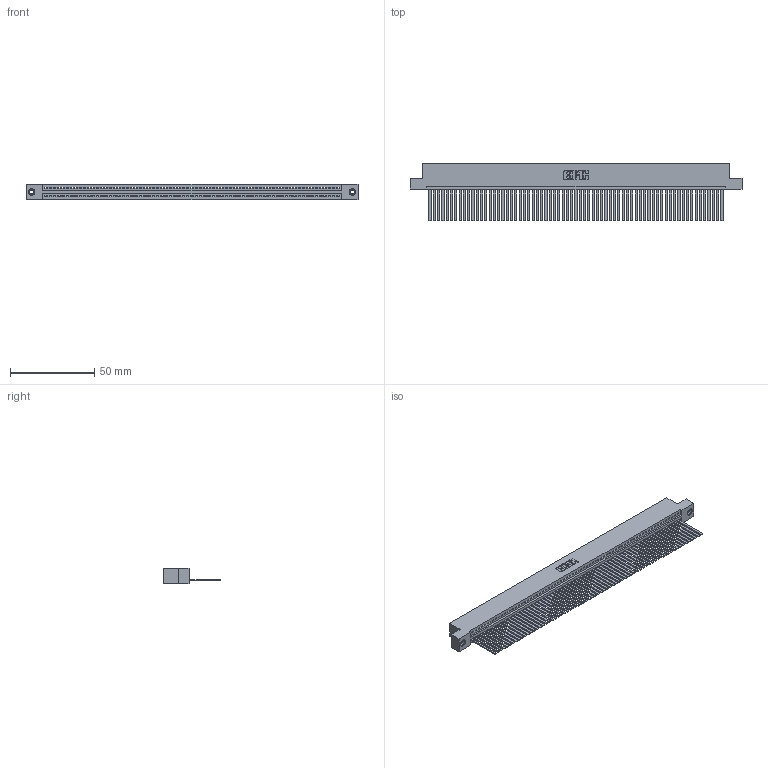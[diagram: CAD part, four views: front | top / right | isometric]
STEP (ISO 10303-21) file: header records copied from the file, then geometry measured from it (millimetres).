
FILE_DESCRIPTION (( 'STEP AP203' ), '1' );
FILE_NAME ('345-069-544-108.STEP', '2018-09-30T19:56:13', ( '' ), ( '' ), 'SwSTEP 2.0', 'SolidWorks 2016', '' );
FILE_SCHEMA (( 'CONFIG_CONTROL_DESIGN' ));
Length unit declared in the file: inch
Products named in the file (4): 345 Part_Flush Mounting Lugs - 0.156 Dia-TI; 345-250-001_345-250-003-102; 345-292-001_345-293-144; 345-069-544-108
Assembly tree (72 placements, depth 2):
  345-069-544-108
    345 Part_Flush Mounting Lugs - 0.156 Dia-TI
    345-292-001_345-293-144  x69
    345-250-001_345-250-003-102  x2
Bounding box: 196.47 x 33.96 x 9.4 mm (x, y, z)
Volume: 19674.6 mm3; surface area: 28930.9 mm2
Topology: 72 solids, 72 shells, 3774 faces, 11379 edges, 7486 vertices
Faces by surface type: plane 2596, cylinder 1162, cone 12, torus 4
Entity records: 49298 total; most frequent: CARTESIAN_POINT 8518, ORIENTED_EDGE 8514, DIRECTION 7425, EDGE_CURVE 4257, LINE 3833, VECTOR 3833, VERTEX_POINT 2832, AXIS2_PLACEMENT_3D 1796
